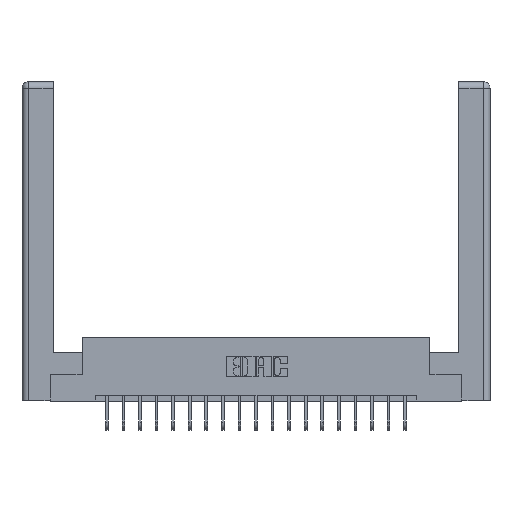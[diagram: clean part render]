
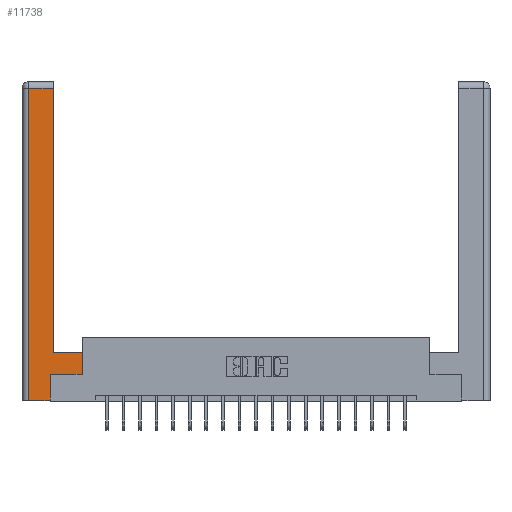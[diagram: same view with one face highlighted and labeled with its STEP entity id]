
A CAD part, top view. The second image highlights one B-rep face of the part: STEP entity #11738.
In plain terms, the highlighted planar face has unit normal (0, 0, 1).
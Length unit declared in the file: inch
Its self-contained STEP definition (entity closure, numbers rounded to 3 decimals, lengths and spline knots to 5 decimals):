
#396 = VERTEX_POINT ( 'NONE', #17761 ) ;
#642 = CARTESIAN_POINT ( 'NONE',  ( 0., 0., 0. ) ) ;
#1031 = EDGE_CURVE ( 'NONE', #12065, #5632, #13919, .T. ) ;
#1045 = ORIENTED_EDGE ( 'NONE', *, *, #14247, .T. ) ;
#1318 = VERTEX_POINT ( 'NONE', #2005 ) ;
#1630 = CARTESIAN_POINT ( 'NONE',  ( 0.265, 0.245, 0. ) ) ;
#1680 = CARTESIAN_POINT ( 'NONE',  ( 0.0615, 0., 0. ) ) ;
#1920 = LINE ( 'NONE', #11122, #19139 ) ;
#2005 = CARTESIAN_POINT ( 'NONE',  ( 0.0615, 0., 0. ) ) ;
#2169 = DIRECTION ( 'NONE',  ( -1., 0., 0. ) ) ;
#2338 = VECTOR ( 'NONE', #5797, 39.37008 ) ;
#2753 = EDGE_CURVE ( 'NONE', #11942, #9575, #4589, .T. ) ;
#2850 = CARTESIAN_POINT ( 'NONE',  ( 0.0615, 2.94, 0. ) ) ;
#3203 = CARTESIAN_POINT ( 'NONE',  ( 0.265, 0., 0. ) ) ;
#3602 = PLANE ( 'NONE',  #4034 ) ;
#3638 = FACE_OUTER_BOUND ( 'NONE', #4833, .T. ) ;
#3812 = VECTOR ( 'NONE', #17927, 39.37008 ) ;
#3969 = EDGE_CURVE ( 'NONE', #11269, #1318, #15256, .T. ) ;
#3979 = EDGE_CURVE ( 'NONE', #1318, #11942, #19830, .T. ) ;
#4034 = AXIS2_PLACEMENT_3D ( 'NONE', #642, #15795, #2169 ) ;
#4589 = LINE ( 'NONE', #5366, #13644 ) ;
#4833 = EDGE_LOOP ( 'NONE', ( #18436, #5841, #11081, #17399, #10052, #5406, #8766, #1045 ) ) ;
#5366 = CARTESIAN_POINT ( 'NONE',  ( 0.265, 0.245, 0. ) ) ;
#5372 = DIRECTION ( 'NONE',  ( 0., 1., 0. ) ) ;
#5406 = ORIENTED_EDGE ( 'NONE', *, *, #17535, .T. ) ;
#5632 = VERTEX_POINT ( 'NONE', #13374 ) ;
#5797 = DIRECTION ( 'NONE',  ( 0., 1., 0. ) ) ;
#5841 = ORIENTED_EDGE ( 'NONE', *, *, #11794, .T. ) ;
#5961 = CARTESIAN_POINT ( 'NONE',  ( 0.0615, 2.94, 0. ) ) ;
#6194 = CARTESIAN_POINT ( 'NONE',  ( 0.265, 0., 0. ) ) ;
#7047 = CARTESIAN_POINT ( 'NONE',  ( 0.295, 2.94, 0. ) ) ;
#7270 = VECTOR ( 'NONE', #5372, 39.37008 ) ;
#7918 = DIRECTION ( 'NONE',  ( 0., -1., 0. ) ) ;
#8766 = ORIENTED_EDGE ( 'NONE', *, *, #1031, .T. ) ;
#9288 = LINE ( 'NONE', #14919, #2338 ) ;
#9575 = VERTEX_POINT ( 'NONE', #1630 ) ;
#10052 = ORIENTED_EDGE ( 'NONE', *, *, #2753, .T. ) ;
#11081 = ORIENTED_EDGE ( 'NONE', *, *, #3969, .T. ) ;
#11122 = CARTESIAN_POINT ( 'NONE',  ( 0.565, 0.245, 0. ) ) ;
#11256 = CARTESIAN_POINT ( 'NONE',  ( 0.565, 0.245, 0. ) ) ;
#11269 = VERTEX_POINT ( 'NONE', #2850 ) ;
#11373 = DIRECTION ( 'NONE',  ( 1., 0., 0. ) ) ;
#11425 = DIRECTION ( 'NONE',  ( 0., 1., 0. ) ) ;
#11738 = ADVANCED_FACE ( 'NONE', ( #3638 ), #3602, .F. ) ;
#11794 = EDGE_CURVE ( 'NONE', #18585, #11269, #17697, .T. ) ;
#11942 = VERTEX_POINT ( 'NONE', #3203 ) ;
#12065 = VERTEX_POINT ( 'NONE', #11256 ) ;
#12403 = LINE ( 'NONE', #16264, #3812 ) ;
#13339 = CARTESIAN_POINT ( 'NONE',  ( 0.565, 0.45, 0. ) ) ;
#13374 = CARTESIAN_POINT ( 'NONE',  ( 0.565, 0.45, 0. ) ) ;
#13636 = VECTOR ( 'NONE', #19378, 39.37008 ) ;
#13644 = VECTOR ( 'NONE', #11425, 39.37008 ) ;
#13919 = LINE ( 'NONE', #13339, #7270 ) ;
#14247 = EDGE_CURVE ( 'NONE', #5632, #396, #12403, .T. ) ;
#14409 = EDGE_CURVE ( 'NONE', #396, #18585, #9288, .T. ) ;
#14919 = CARTESIAN_POINT ( 'NONE',  ( 0.295, 3., 0. ) ) ;
#15256 = LINE ( 'NONE', #1680, #16691 ) ;
#15511 = VECTOR ( 'NONE', #11373, 39.37008 ) ;
#15707 = DIRECTION ( 'NONE',  ( 1., 0., 0. ) ) ;
#15795 = DIRECTION ( 'NONE',  ( 0., 0., -1. ) ) ;
#16264 = CARTESIAN_POINT ( 'NONE',  ( 0.295, 0.45, 0. ) ) ;
#16691 = VECTOR ( 'NONE', #7918, 39.37008 ) ;
#17399 = ORIENTED_EDGE ( 'NONE', *, *, #3979, .T. ) ;
#17535 = EDGE_CURVE ( 'NONE', #9575, #12065, #1920, .T. ) ;
#17697 = LINE ( 'NONE', #5961, #13636 ) ;
#17761 = CARTESIAN_POINT ( 'NONE',  ( 0.295, 0.45, 0. ) ) ;
#17927 = DIRECTION ( 'NONE',  ( -1., 0., 0. ) ) ;
#18436 = ORIENTED_EDGE ( 'NONE', *, *, #14409, .T. ) ;
#18585 = VERTEX_POINT ( 'NONE', #7047 ) ;
#19139 = VECTOR ( 'NONE', #15707, 39.37008 ) ;
#19378 = DIRECTION ( 'NONE',  ( -1., 0., 0. ) ) ;
#19830 = LINE ( 'NONE', #6194, #15511 ) ;
